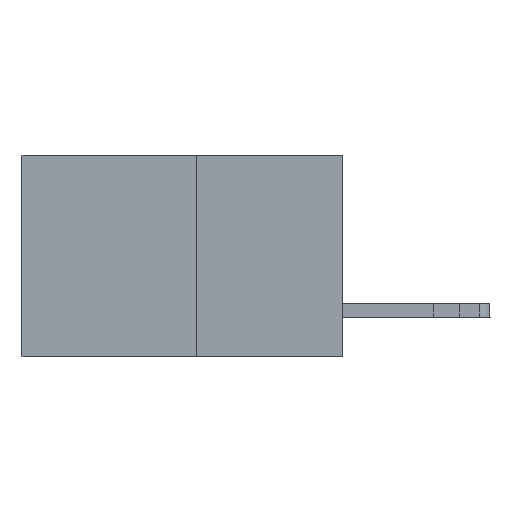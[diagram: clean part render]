
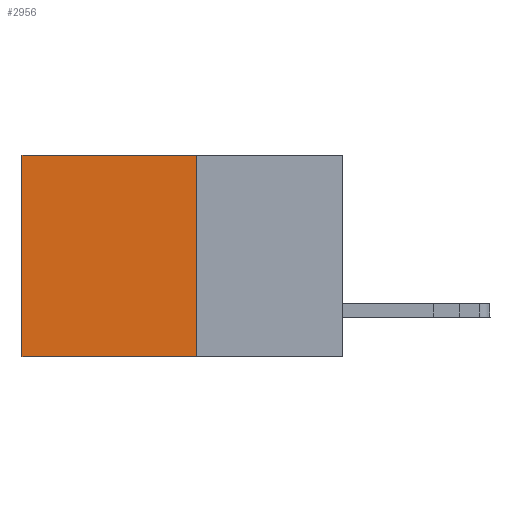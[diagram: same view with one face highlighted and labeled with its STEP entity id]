
A CAD part, left-side view. The second image highlights one B-rep face of the part: STEP entity #2956.
In plain terms, the highlighted planar face has unit normal (-1, 0, 0).
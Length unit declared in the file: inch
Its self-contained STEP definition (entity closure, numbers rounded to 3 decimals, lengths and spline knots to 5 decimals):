
#433 = EDGE_LOOP ( 'NONE', ( #14917, #4088, #7916, #16031 ) ) ;
#1002 = DIRECTION ( 'NONE',  ( 0., 0., -1. ) ) ;
#1571 = VERTEX_POINT ( 'NONE', #9860 ) ;
#2956 = ADVANCED_FACE ( 'NONE', ( #6835 ), #4845, .F. ) ;
#4088 = ORIENTED_EDGE ( 'NONE', *, *, #10631, .F. ) ;
#4739 = VERTEX_POINT ( 'NONE', #10102 ) ;
#4845 = PLANE ( 'NONE',  #21456 ) ;
#6120 = CARTESIAN_POINT ( 'NONE',  ( 0.277, 0.27, -0.37 ) ) ;
#6679 = LINE ( 'NONE', #11807, #18176 ) ;
#6773 = CARTESIAN_POINT ( 'NONE',  ( 0.277, 0.27, -0.37 ) ) ;
#6835 = FACE_OUTER_BOUND ( 'NONE', #433, .T. ) ;
#7213 = CARTESIAN_POINT ( 'NONE',  ( 0.277, 0.59, -0.37 ) ) ;
#7916 = ORIENTED_EDGE ( 'NONE', *, *, #12638, .F. ) ;
#9860 = CARTESIAN_POINT ( 'NONE',  ( 0.277, 0.59, -0.37 ) ) ;
#9869 = CARTESIAN_POINT ( 'NONE',  ( 0.277, 0.27, -0.37 ) ) ;
#10102 = CARTESIAN_POINT ( 'NONE',  ( 0.277, 0.59, 0. ) ) ;
#10349 = VECTOR ( 'NONE', #14314, 39.37008 ) ;
#10631 = EDGE_CURVE ( 'NONE', #21205, #1571, #14417, .T. ) ;
#10705 = LINE ( 'NONE', #7213, #10349 ) ;
#11807 = CARTESIAN_POINT ( 'NONE',  ( 0.277, 0.27, 0. ) ) ;
#12150 = EDGE_CURVE ( 'NONE', #15784, #4739, #6679, .T. ) ;
#12638 = EDGE_CURVE ( 'NONE', #15784, #21205, #19240, .T. ) ;
#13641 = VECTOR ( 'NONE', #21902, 39.37008 ) ;
#13891 = EDGE_CURVE ( 'NONE', #4739, #1571, #10705, .T. ) ;
#14314 = DIRECTION ( 'NONE',  ( 0., 0., -1. ) ) ;
#14417 = LINE ( 'NONE', #21776, #13641 ) ;
#14917 = ORIENTED_EDGE ( 'NONE', *, *, #13891, .T. ) ;
#15514 = VECTOR ( 'NONE', #19020, 39.37008 ) ;
#15784 = VERTEX_POINT ( 'NONE', #16640 ) ;
#16031 = ORIENTED_EDGE ( 'NONE', *, *, #12150, .T. ) ;
#16640 = CARTESIAN_POINT ( 'NONE',  ( 0.277, 0.27, 0. ) ) ;
#16976 = DIRECTION ( 'NONE',  ( 1., 0., 0. ) ) ;
#18176 = VECTOR ( 'NONE', #22790, 39.37008 ) ;
#19020 = DIRECTION ( 'NONE',  ( 0., 0., -1. ) ) ;
#19240 = LINE ( 'NONE', #6773, #15514 ) ;
#21205 = VERTEX_POINT ( 'NONE', #6120 ) ;
#21456 = AXIS2_PLACEMENT_3D ( 'NONE', #9869, #16976, #1002 ) ;
#21776 = CARTESIAN_POINT ( 'NONE',  ( 0.277, 0.27, -0.37 ) ) ;
#21902 = DIRECTION ( 'NONE',  ( 0., 1., 0. ) ) ;
#22790 = DIRECTION ( 'NONE',  ( 0., 1., 0. ) ) ;
